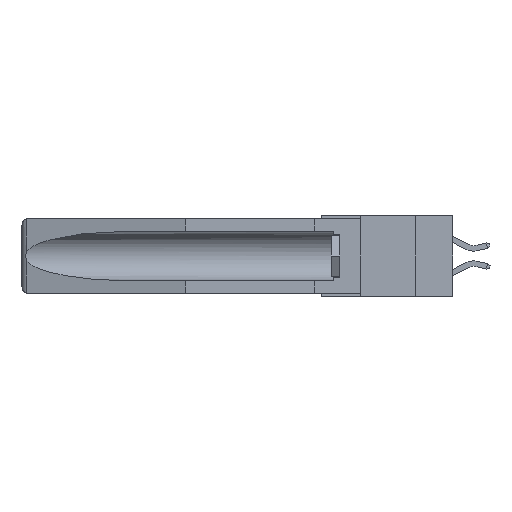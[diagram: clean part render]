
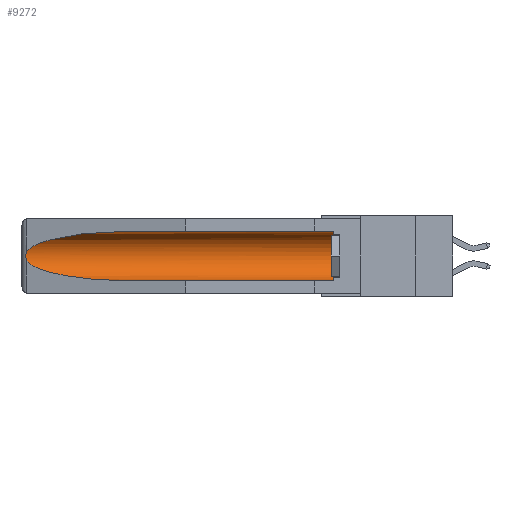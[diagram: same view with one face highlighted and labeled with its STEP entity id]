
A CAD part, left-side view. The second image highlights one B-rep face of the part: STEP entity #9272.
In plain terms, the highlighted cylindrical face has radius 2.857 mm (diameter 5.715 mm), a partial arc.
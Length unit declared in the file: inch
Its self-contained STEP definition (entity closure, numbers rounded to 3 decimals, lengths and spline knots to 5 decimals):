
#408 = CARTESIAN_POINT ( 'NONE',  ( 0.26537, 1.52718, -0.14972 ) ) ;
#1387 = EDGE_CURVE ( 'NONE', #8925, #14607, #13641, .T. ) ;
#1526 = ORIENTED_EDGE ( 'NONE', *, *, #12304, .T. ) ;
#2058 = CARTESIAN_POINT ( 'NONE',  ( 0.21114, 1.30732, -0.059 ) ) ;
#2119 = B_SPLINE_CURVE_WITH_KNOTS ( 'NONE', 3,
 ( #408, #10734, #12030, #13165, #14580, #6756, #9418, #14642, #15945, #6934 ),
 .UNSPECIFIED., .F., .F.,
 ( 4, 2, 2, 2, 4 ),
 ( 0., 0.00029, 0.00058, 0.00087, 0.00117 ),
 .UNSPECIFIED. ) ;
#2551 = CARTESIAN_POINT ( 'NONE',  ( 0.155, 1.07973, -0.284 ) ) ;
#2573 = EDGE_CURVE ( 'NONE', #11012, #10264, #6686, .T. ) ;
#2602 = VERTEX_POINT ( 'NONE', #13873 ) ;
#3285 = CARTESIAN_POINT ( 'NONE',  ( 0.155, -0.30754, -0.284 ) ) ;
#3332 = CARTESIAN_POINT ( 'NONE',  ( 0.25451, 1.48313, -0.09465 ) ) ;
#5059 = EDGE_CURVE ( 'NONE', #2602, #14607, #6161, .T. ) ;
#5272 = AXIS2_PLACEMENT_3D ( 'NONE', #8244, #16026, #8345 ) ;
#6037 = ORIENTED_EDGE ( 'NONE', *, *, #1387, .F. ) ;
#6161 =( BOUNDED_CURVE ( )  B_SPLINE_CURVE ( 3, ( #12207, #15103, #7310, #16293 ),
 .UNSPECIFIED., .F., .F. ) 
 B_SPLINE_CURVE_WITH_KNOTS ( ( 4, 4 ),
 ( 0.1948, 1.5708 ),
 .UNSPECIFIED. ) 
 CURVE ( )  GEOMETRIC_REPRESENTATION_ITEM ( )  RATIONAL_B_SPLINE_CURVE ( ( 1., 0.848, 0.848, 1. ) ) 
 REPRESENTATION_ITEM ( '' )  );
#6340 = CARTESIAN_POINT ( 'NONE',  ( 0.155, 1.07973, -0.059 ) ) ;
#6686 =( BOUNDED_CURVE ( )  B_SPLINE_CURVE ( 3, ( #16195, #2058, #3332, #12822 ),
 .UNSPECIFIED., .F., .F. ) 
 B_SPLINE_CURVE_WITH_KNOTS ( ( 4, 4 ),
 ( 4.71239, 6.08839 ),
 .UNSPECIFIED. ) 
 CURVE ( )  GEOMETRIC_REPRESENTATION_ITEM ( )  RATIONAL_B_SPLINE_CURVE ( ( 1., 0.848, 0.848, 1. ) ) 
 REPRESENTATION_ITEM ( '' )  );
#6756 = CARTESIAN_POINT ( 'NONE',  ( 0.2675, 1.53308, -0.17534 ) ) ;
#6934 = CARTESIAN_POINT ( 'NONE',  ( 0.26537, 1.52718, -0.19328 ) ) ;
#6992 = CARTESIAN_POINT ( 'NONE',  ( 0.155, 0.126, -0.284 ) ) ;
#7310 = CARTESIAN_POINT ( 'NONE',  ( 0.21114, 1.30732, -0.284 ) ) ;
#7592 = CARTESIAN_POINT ( 'NONE',  ( 0.155, -0.30754, -0.059 ) ) ;
#7682 = AXIS2_PLACEMENT_3D ( 'NONE', #12756, #11568, #15458 ) ;
#8244 = CARTESIAN_POINT ( 'NONE',  ( 0.155, 0.126, -0.1715 ) ) ;
#8345 = DIRECTION ( 'NONE',  ( 0., 0., 1. ) ) ;
#8635 = EDGE_CURVE ( 'NONE', #16042, #11012, #13648, .T. ) ;
#8925 = VERTEX_POINT ( 'NONE', #6992 ) ;
#9272 = ADVANCED_FACE ( 'NONE', ( #9797 ), #10192, .F. ) ;
#9418 = CARTESIAN_POINT ( 'NONE',  ( 0.2673, 1.53269, -0.17917 ) ) ;
#9426 = VECTOR ( 'NONE', #16036, 39.37008 ) ;
#9797 = FACE_OUTER_BOUND ( 'NONE', #14100, .T. ) ;
#10043 = ORIENTED_EDGE ( 'NONE', *, *, #14375, .T. ) ;
#10102 = CARTESIAN_POINT ( 'NONE',  ( 0.155, 0.126, -0.059 ) ) ;
#10192 = CYLINDRICAL_SURFACE ( 'NONE', #7682, 0.1125 ) ;
#10264 = VERTEX_POINT ( 'NONE', #12318 ) ;
#10330 = DIRECTION ( 'NONE',  ( 0., 1., 0. ) ) ;
#10700 = CIRCLE ( 'NONE', #5272, 0.1125 ) ;
#10734 = CARTESIAN_POINT ( 'NONE',  ( 0.26597, 1.52961, -0.15275 ) ) ;
#10866 = ORIENTED_EDGE ( 'NONE', *, *, #2573, .T. ) ;
#11012 = VERTEX_POINT ( 'NONE', #6340 ) ;
#11027 = ORIENTED_EDGE ( 'NONE', *, *, #5059, .T. ) ;
#11568 = DIRECTION ( 'NONE',  ( 0., 1., 0. ) ) ;
#12030 = CARTESIAN_POINT ( 'NONE',  ( 0.26654, 1.53092, -0.15636 ) ) ;
#12207 = CARTESIAN_POINT ( 'NONE',  ( 0.26537, 1.52718, -0.19328 ) ) ;
#12304 = EDGE_CURVE ( 'NONE', #8925, #16042, #10700, .T. ) ;
#12318 = CARTESIAN_POINT ( 'NONE',  ( 0.26537, 1.52718, -0.14972 ) ) ;
#12756 = CARTESIAN_POINT ( 'NONE',  ( 0.155, -0.30754, -0.1715 ) ) ;
#12822 = CARTESIAN_POINT ( 'NONE',  ( 0.26537, 1.52718, -0.14972 ) ) ;
#13165 = CARTESIAN_POINT ( 'NONE',  ( 0.2673, 1.5327, -0.16383 ) ) ;
#13641 = LINE ( 'NONE', #3285, #9426 ) ;
#13648 = LINE ( 'NONE', #7592, #15630 ) ;
#13873 = CARTESIAN_POINT ( 'NONE',  ( 0.26537, 1.52718, -0.19328 ) ) ;
#14100 = EDGE_LOOP ( 'NONE', ( #10866, #10043, #11027, #6037, #1526, #15099 ) ) ;
#14375 = EDGE_CURVE ( 'NONE', #10264, #2602, #2119, .T. ) ;
#14580 = CARTESIAN_POINT ( 'NONE',  ( 0.2675, 1.53308, -0.16763 ) ) ;
#14607 = VERTEX_POINT ( 'NONE', #2551 ) ;
#14642 = CARTESIAN_POINT ( 'NONE',  ( 0.26655, 1.53094, -0.18657 ) ) ;
#15099 = ORIENTED_EDGE ( 'NONE', *, *, #8635, .T. ) ;
#15103 = CARTESIAN_POINT ( 'NONE',  ( 0.25451, 1.48313, -0.24835 ) ) ;
#15458 = DIRECTION ( 'NONE',  ( 0., 0., 1. ) ) ;
#15630 = VECTOR ( 'NONE', #10330, 39.37008 ) ;
#15945 = CARTESIAN_POINT ( 'NONE',  ( 0.26597, 1.5296, -0.19026 ) ) ;
#16026 = DIRECTION ( 'NONE',  ( 0., -1., 0. ) ) ;
#16036 = DIRECTION ( 'NONE',  ( 0., 1., 0. ) ) ;
#16042 = VERTEX_POINT ( 'NONE', #10102 ) ;
#16195 = CARTESIAN_POINT ( 'NONE',  ( 0.155, 1.07973, -0.059 ) ) ;
#16293 = CARTESIAN_POINT ( 'NONE',  ( 0.155, 1.07973, -0.284 ) ) ;
